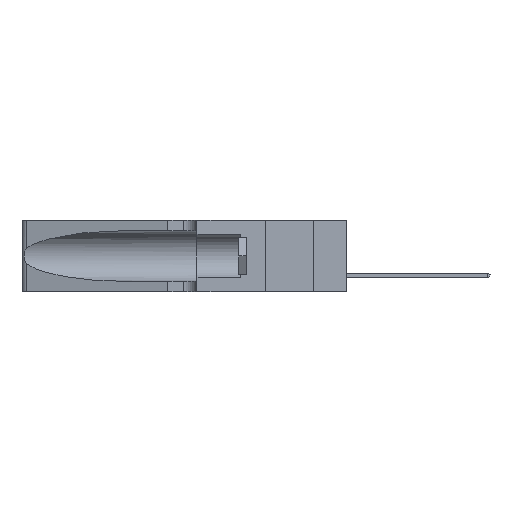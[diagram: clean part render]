
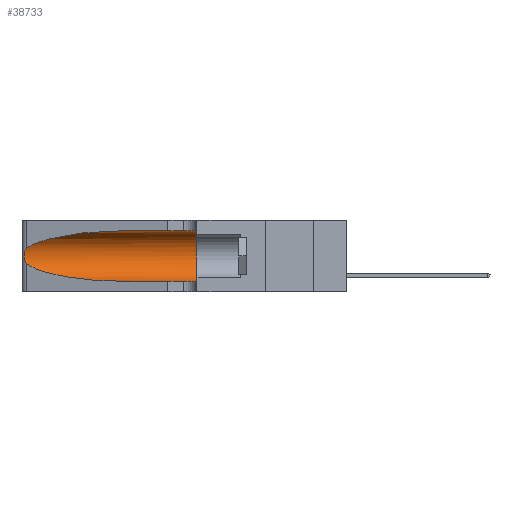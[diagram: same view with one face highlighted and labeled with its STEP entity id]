
A CAD part, left-side view. The second image highlights one B-rep face of the part: STEP entity #38733.
In plain terms, the highlighted cylindrical face has radius 3.308 mm (diameter 6.617 mm), a partial arc.
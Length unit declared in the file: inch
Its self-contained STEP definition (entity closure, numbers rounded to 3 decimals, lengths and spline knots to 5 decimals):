
#910 = CARTESIAN_POINT ( 'NONE',  ( 0.1305, 1.61858, 0.185 ) ) ;
#1890 =( BOUNDED_CURVE ( )  B_SPLINE_CURVE ( 3, ( #27943, #4879, #30981, #31420 ),
 .UNSPECIFIED., .F., .F. ) 
 B_SPLINE_CURVE_WITH_KNOTS ( ( 4, 4 ),
 ( 3.44316, 4.71239 ),
 .UNSPECIFIED. ) 
 CURVE ( )  GEOMETRIC_REPRESENTATION_ITEM ( )  RATIONAL_B_SPLINE_CURVE ( ( 1., 0.87, 0.87, 1. ) ) 
 REPRESENTATION_ITEM ( '' )  );
#2292 = EDGE_CURVE ( 'NONE', #10237, #17822, #15742, .T. ) ;
#2374 = EDGE_CURVE ( 'NONE', #6131, #14734, #24184, .T. ) ;
#2590 = DIRECTION ( 'NONE',  ( 0., -1., 0. ) ) ;
#2698 = ORIENTED_EDGE ( 'NONE', *, *, #2292, .T. ) ;
#3849 = CARTESIAN_POINT ( 'NONE',  ( 0.25555, 1.22993, 0.14849 ) ) ;
#4473 = EDGE_CURVE ( 'NONE', #10237, #30890, #37871, .T. ) ;
#4879 = CARTESIAN_POINT ( 'NONE',  ( 0.2373, 1.15595, 0.08982 ) ) ;
#4960 = CARTESIAN_POINT ( 'NONE',  ( 0.18966, 0.96281, 0.31525 ) ) ;
#4971 = CARTESIAN_POINT ( 'NONE',  ( 0.1305, 0.72297, 0.31525 ) ) ;
#6131 = VERTEX_POINT ( 'NONE', #40628 ) ;
#6256 = ORIENTED_EDGE ( 'NONE', *, *, #4473, .F. ) ;
#6516 = DIRECTION ( 'NONE',  ( 0., -1., 0. ) ) ;
#7134 = CARTESIAN_POINT ( 'NONE',  ( 0.25487, 1.22718, 0.14631 ) ) ;
#9035 = CARTESIAN_POINT ( 'NONE',  ( 0.1305, 1.61858, 0.31525 ) ) ;
#9841 = CARTESIAN_POINT ( 'NONE',  ( 0.1305, 0.35, 0.31525 ) ) ;
#10237 = VERTEX_POINT ( 'NONE', #4971 ) ;
#10858 = CARTESIAN_POINT ( 'NONE',  ( 0.25639, 1.23184, 0.21858 ) ) ;
#11083 = DIRECTION ( 'NONE',  ( 0., -1., 0. ) ) ;
#13648 = VERTEX_POINT ( 'NONE', #22597 ) ;
#14734 = VERTEX_POINT ( 'NONE', #24610 ) ;
#15371 = ORIENTED_EDGE ( 'NONE', *, *, #31552, .F. ) ;
#15742 =( BOUNDED_CURVE ( )  B_SPLINE_CURVE ( 3, ( #24543, #4960, #24689, #19014 ),
 .UNSPECIFIED., .F., .F. ) 
 B_SPLINE_CURVE_WITH_KNOTS ( ( 4, 4 ),
 ( 1.5708, 2.84003 ),
 .UNSPECIFIED. ) 
 CURVE ( )  GEOMETRIC_REPRESENTATION_ITEM ( )  RATIONAL_B_SPLINE_CURVE ( ( 1., 0.87, 0.87, 1. ) ) 
 REPRESENTATION_ITEM ( '' )  );
#16843 = CARTESIAN_POINT ( 'NONE',  ( 0.25789, 1.23486, 0.15765 ) ) ;
#17125 = CARTESIAN_POINT ( 'NONE',  ( 0.25787, 1.23484, 0.2124 ) ) ;
#17431 = CARTESIAN_POINT ( 'NONE',  ( 0.25856, 1.23593, 0.16098 ) ) ;
#17822 = VERTEX_POINT ( 'NONE', #21747 ) ;
#17990 = CIRCLE ( 'NONE', #35168, 0.13025 ) ;
#18012 = AXIS2_PLACEMENT_3D ( 'NONE', #910, #11083, #20926 ) ;
#18831 = EDGE_LOOP ( 'NONE', ( #2698, #34852, #29305, #32300, #15371, #6256 ) ) ;
#19014 = CARTESIAN_POINT ( 'NONE',  ( 0.25487, 1.22718, 0.22369 ) ) ;
#19468 = CARTESIAN_POINT ( 'NONE',  ( 0.1305, 0.35, 0.185 ) ) ;
#20282 = CARTESIAN_POINT ( 'NONE',  ( 0.26018, 1.23835, 0.19895 ) ) ;
#20419 = CARTESIAN_POINT ( 'NONE',  ( 0.26075, 1.23896, 0.19203 ) ) ;
#20926 = DIRECTION ( 'NONE',  ( 0., 0., -1. ) ) ;
#21489 = EDGE_CURVE ( 'NONE', #13648, #6131, #1890, .T. ) ;
#21747 = CARTESIAN_POINT ( 'NONE',  ( 0.25487, 1.22718, 0.22369 ) ) ;
#22168 = VECTOR ( 'NONE', #6516, 39.37008 ) ;
#22597 = CARTESIAN_POINT ( 'NONE',  ( 0.25487, 1.22718, 0.14631 ) ) ;
#23436 = CARTESIAN_POINT ( 'NONE',  ( 0.25639, 1.23186, 0.15144 ) ) ;
#24184 = LINE ( 'NONE', #39280, #22168 ) ;
#24430 = EDGE_CURVE ( 'NONE', #17822, #13648, #36693, .T. ) ;
#24543 = CARTESIAN_POINT ( 'NONE',  ( 0.1305, 0.72297, 0.31525 ) ) ;
#24610 = CARTESIAN_POINT ( 'NONE',  ( 0.1305, 0.35, 0.05475 ) ) ;
#24689 = CARTESIAN_POINT ( 'NONE',  ( 0.2373, 1.15595, 0.28018 ) ) ;
#25597 = VECTOR ( 'NONE', #2590, 39.37008 ) ;
#27150 = CYLINDRICAL_SURFACE ( 'NONE', #18012, 0.13025 ) ;
#27943 = CARTESIAN_POINT ( 'NONE',  ( 0.25487, 1.22718, 0.14631 ) ) ;
#29305 = ORIENTED_EDGE ( 'NONE', *, *, #21489, .T. ) ;
#29971 = CARTESIAN_POINT ( 'NONE',  ( 0.25555, 1.22994, 0.2215 ) ) ;
#30890 = VERTEX_POINT ( 'NONE', #9841 ) ;
#30981 = CARTESIAN_POINT ( 'NONE',  ( 0.18966, 0.96281, 0.05475 ) ) ;
#31420 = CARTESIAN_POINT ( 'NONE',  ( 0.1305, 0.72297, 0.05475 ) ) ;
#31552 = EDGE_CURVE ( 'NONE', #30890, #14734, #17990, .T. ) ;
#32300 = ORIENTED_EDGE ( 'NONE', *, *, #2374, .T. ) ;
#33766 = CARTESIAN_POINT ( 'NONE',  ( 0.26075, 1.23896, 0.178 ) ) ;
#34852 = ORIENTED_EDGE ( 'NONE', *, *, #24430, .T. ) ;
#35168 = AXIS2_PLACEMENT_3D ( 'NONE', #19468, #38843, #35556 ) ;
#35556 = DIRECTION ( 'NONE',  ( 0., 0., 1. ) ) ;
#35850 = FACE_OUTER_BOUND ( 'NONE', #18831, .T. ) ;
#36693 = B_SPLINE_CURVE_WITH_KNOTS ( 'NONE', 3,
 ( #36893, #29971, #10858, #17125, #40042, #20282, #20419, #33766, #37042, #17431, #16843, #23436, #3849, #7134 ),
 .UNSPECIFIED., .F., .F.,
 ( 4, 2, 2, 2, 2, 2, 4 ),
 ( 0., 0.00027, 0.00053, 0.00107, 0.0016, 0.00187, 0.00214 ),
 .UNSPECIFIED. ) ;
#36893 = CARTESIAN_POINT ( 'NONE',  ( 0.25487, 1.22718, 0.22369 ) ) ;
#37042 = CARTESIAN_POINT ( 'NONE',  ( 0.26017, 1.23833, 0.17102 ) ) ;
#37871 = LINE ( 'NONE', #9035, #25597 ) ;
#38733 = ADVANCED_FACE ( 'NONE', ( #35850 ), #27150, .F. ) ;
#38843 = DIRECTION ( 'NONE',  ( 0., 1., 0. ) ) ;
#39280 = CARTESIAN_POINT ( 'NONE',  ( 0.1305, 1.61858, 0.05475 ) ) ;
#40042 = CARTESIAN_POINT ( 'NONE',  ( 0.25854, 1.2359, 0.20912 ) ) ;
#40628 = CARTESIAN_POINT ( 'NONE',  ( 0.1305, 0.72297, 0.05475 ) ) ;
